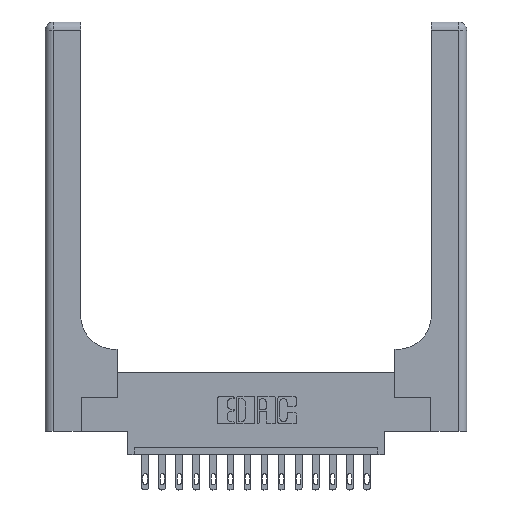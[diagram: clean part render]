
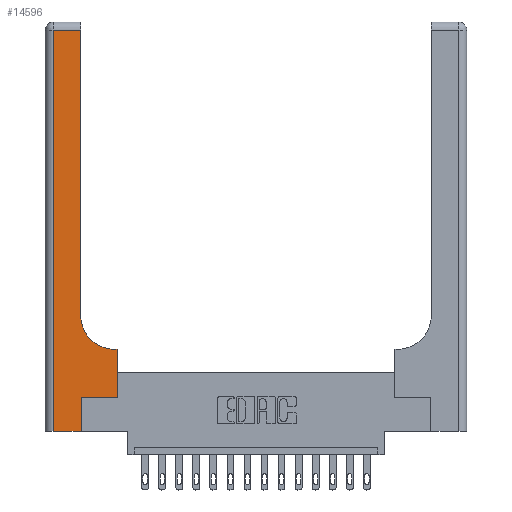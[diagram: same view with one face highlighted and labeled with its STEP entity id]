
A CAD part, top view. The second image highlights one B-rep face of the part: STEP entity #14596.
In plain terms, the highlighted planar face has unit normal (0, 0, 1).
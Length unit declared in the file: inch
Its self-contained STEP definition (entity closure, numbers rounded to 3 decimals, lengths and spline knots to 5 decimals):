
#111 = DIRECTION ( 'NONE',  ( 1., 0., 0. ) ) ;
#831 = CARTESIAN_POINT ( 'NONE',  ( 0.06, 3., 0.37 ) ) ;
#922 = LINE ( 'NONE', #2397, #16388 ) ;
#1089 = DIRECTION ( 'NONE',  ( 0., -1., 0. ) ) ;
#1129 = AXIS2_PLACEMENT_3D ( 'NONE', #5920, #11480, #111 ) ;
#1730 = EDGE_CURVE ( 'NONE', #8984, #10809, #16544, .T. ) ;
#1826 = VERTEX_POINT ( 'NONE', #7130 ) ;
#2287 = CARTESIAN_POINT ( 'NONE',  ( 0.51, 0.6, 0.37 ) ) ;
#2397 = CARTESIAN_POINT ( 'NONE',  ( 0., 2.94, 0.37 ) ) ;
#2426 = PLANE ( 'NONE',  #11931 ) ;
#2456 = VECTOR ( 'NONE', #2799, 39.37008 ) ;
#2710 = ORIENTED_EDGE ( 'NONE', *, *, #17863, .T. ) ;
#2722 = CARTESIAN_POINT ( 'NONE',  ( 0.06, 2.94, 0.37 ) ) ;
#2799 = DIRECTION ( 'NONE',  ( 0., 1., 0. ) ) ;
#2801 = VECTOR ( 'NONE', #1089, 39.37008 ) ;
#2853 = CARTESIAN_POINT ( 'NONE',  ( 0.06, 0., 0.37 ) ) ;
#3152 = VERTEX_POINT ( 'NONE', #2287 ) ;
#3194 = CARTESIAN_POINT ( 'NONE',  ( 0.265, 0.25, 0.37 ) ) ;
#3328 = ORIENTED_EDGE ( 'NONE', *, *, #9790, .T. ) ;
#3684 = LINE ( 'NONE', #7891, #13950 ) ;
#3702 = LINE ( 'NONE', #14673, #13966 ) ;
#3724 = VERTEX_POINT ( 'NONE', #11198 ) ;
#3909 = FACE_OUTER_BOUND ( 'NONE', #14616, .T. ) ;
#4109 = CARTESIAN_POINT ( 'NONE',  ( 0.265, 0., 0.37 ) ) ;
#4274 = CARTESIAN_POINT ( 'NONE',  ( 0.528, 0.6, 0.37 ) ) ;
#4361 = EDGE_CURVE ( 'NONE', #6255, #8629, #6538, .T. ) ;
#5869 = LINE ( 'NONE', #17034, #12538 ) ;
#5920 = CARTESIAN_POINT ( 'NONE',  ( 0.51, 0.85, 0.37 ) ) ;
#6012 = CARTESIAN_POINT ( 'NONE',  ( 0.26, 3., 0.37 ) ) ;
#6255 = VERTEX_POINT ( 'NONE', #2722 ) ;
#6479 = LINE ( 'NONE', #17807, #11632 ) ;
#6538 = LINE ( 'NONE', #831, #2801 ) ;
#7043 = ORIENTED_EDGE ( 'NONE', *, *, #4361, .T. ) ;
#7130 = CARTESIAN_POINT ( 'NONE',  ( 0.26, 2.94, 0.37 ) ) ;
#7230 = EDGE_CURVE ( 'NONE', #8629, #8984, #6479, .T. ) ;
#7532 = DIRECTION ( 'NONE',  ( 1., 0., 0. ) ) ;
#7832 = ORIENTED_EDGE ( 'NONE', *, *, #14889, .T. ) ;
#7891 = CARTESIAN_POINT ( 'NONE',  ( 0.265, 0.25, 0.37 ) ) ;
#7989 = DIRECTION ( 'NONE',  ( -1., 0., 0. ) ) ;
#8286 = DIRECTION ( 'NONE',  ( 0., 0., -1. ) ) ;
#8376 = DIRECTION ( 'NONE',  ( -1., 0., 0. ) ) ;
#8629 = VERTEX_POINT ( 'NONE', #2853 ) ;
#8765 = ORIENTED_EDGE ( 'NONE', *, *, #15724, .T. ) ;
#8802 = ORIENTED_EDGE ( 'NONE', *, *, #1730, .T. ) ;
#8842 = LINE ( 'NONE', #6012, #10493 ) ;
#8984 = VERTEX_POINT ( 'NONE', #9713 ) ;
#9482 = CARTESIAN_POINT ( 'NONE',  ( 0., 3., 0.37 ) ) ;
#9713 = CARTESIAN_POINT ( 'NONE',  ( 0.265, 0., 0.37 ) ) ;
#9790 = EDGE_CURVE ( 'NONE', #1826, #6255, #922, .T. ) ;
#10108 = DIRECTION ( 'NONE',  ( 0., 1., 0. ) ) ;
#10373 = DIRECTION ( 'NONE',  ( 0., 1., 0. ) ) ;
#10493 = VECTOR ( 'NONE', #10108, 39.37008 ) ;
#10809 = VERTEX_POINT ( 'NONE', #3194 ) ;
#11198 = CARTESIAN_POINT ( 'NONE',  ( 0.26, 0.85, 0.37 ) ) ;
#11480 = DIRECTION ( 'NONE',  ( 0., 0., -1. ) ) ;
#11632 = VECTOR ( 'NONE', #15204, 39.37008 ) ;
#11664 = ORIENTED_EDGE ( 'NONE', *, *, #15811, .T. ) ;
#11931 = AXIS2_PLACEMENT_3D ( 'NONE', #9482, #8286, #8376 ) ;
#12332 = VERTEX_POINT ( 'NONE', #4274 ) ;
#12537 = ORIENTED_EDGE ( 'NONE', *, *, #16172, .T. ) ;
#12538 = VECTOR ( 'NONE', #16936, 39.37008 ) ;
#12825 = CIRCLE ( 'NONE', #1129, 0.25 ) ;
#13950 = VECTOR ( 'NONE', #7532, 39.37008 ) ;
#13966 = VECTOR ( 'NONE', #10373, 39.37008 ) ;
#14596 = ADVANCED_FACE ( 'NONE', ( #3909 ), #2426, .F. ) ;
#14616 = EDGE_LOOP ( 'NONE', ( #8765, #3328, #7043, #16476, #8802, #12537, #7832, #2710, #11664 ) ) ;
#14673 = CARTESIAN_POINT ( 'NONE',  ( 0.528, 0.25, 0.37 ) ) ;
#14889 = EDGE_CURVE ( 'NONE', #16421, #12332, #3702, .T. ) ;
#15174 = CARTESIAN_POINT ( 'NONE',  ( 0.528, 0.25, 0.37 ) ) ;
#15204 = DIRECTION ( 'NONE',  ( 1., 0., 0. ) ) ;
#15724 = EDGE_CURVE ( 'NONE', #3724, #1826, #8842, .T. ) ;
#15811 = EDGE_CURVE ( 'NONE', #3152, #3724, #12825, .T. ) ;
#16172 = EDGE_CURVE ( 'NONE', #10809, #16421, #3684, .T. ) ;
#16388 = VECTOR ( 'NONE', #7989, 39.37008 ) ;
#16421 = VERTEX_POINT ( 'NONE', #15174 ) ;
#16476 = ORIENTED_EDGE ( 'NONE', *, *, #7230, .T. ) ;
#16544 = LINE ( 'NONE', #4109, #2456 ) ;
#16936 = DIRECTION ( 'NONE',  ( -1., 0., 0. ) ) ;
#17034 = CARTESIAN_POINT ( 'NONE',  ( 0.26, 0.6, 0.37 ) ) ;
#17807 = CARTESIAN_POINT ( 'NONE',  ( 0., 0., 0.37 ) ) ;
#17863 = EDGE_CURVE ( 'NONE', #12332, #3152, #5869, .T. ) ;
